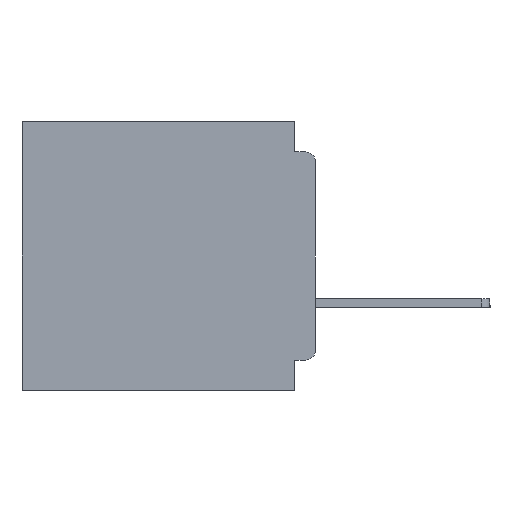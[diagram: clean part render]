
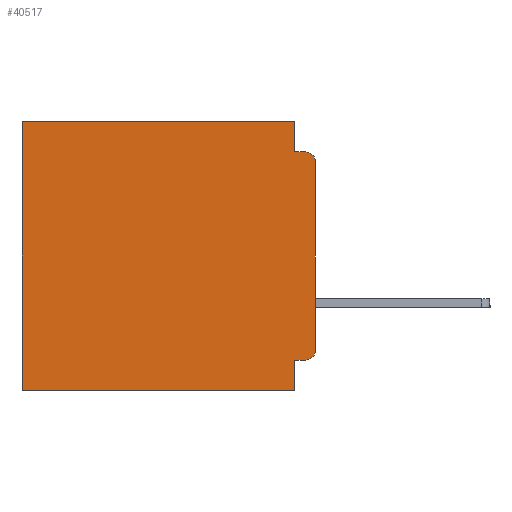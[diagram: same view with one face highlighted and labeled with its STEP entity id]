
A CAD part, left-side view. The second image highlights one B-rep face of the part: STEP entity #40517.
In plain terms, the highlighted planar face has unit normal (-1, 0, 0).
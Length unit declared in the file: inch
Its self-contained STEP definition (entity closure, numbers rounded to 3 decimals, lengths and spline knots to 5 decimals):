
#1040 = ORIENTED_EDGE ( 'NONE', *, *, #40793, .T. ) ;
#1313 = VERTEX_POINT ( 'NONE', #37785 ) ;
#1515 = LINE ( 'NONE', #48837, #16003 ) ;
#2371 = CARTESIAN_POINT ( 'NONE',  ( 0.3, 0.031, -0.4 ) ) ;
#3398 = DIRECTION ( 'NONE',  ( 0., 0., -1. ) ) ;
#3695 = CARTESIAN_POINT ( 'NONE',  ( 0.3, 0., 0. ) ) ;
#3770 = VERTEX_POINT ( 'NONE', #52345 ) ;
#4352 = VECTOR ( 'NONE', #5088, 39.37008 ) ;
#4801 = CARTESIAN_POINT ( 'NONE',  ( 0.3, 0.437, -0.4 ) ) ;
#5088 = DIRECTION ( 'NONE',  ( 0., 0., -1. ) ) ;
#5142 = DIRECTION ( 'NONE',  ( 0., 1., 0. ) ) ;
#5832 = FACE_OUTER_BOUND ( 'NONE', #31797, .T. ) ;
#6410 = VERTEX_POINT ( 'NONE', #62724 ) ;
#6475 = EDGE_CURVE ( 'NONE', #6410, #33333, #1515, .T. ) ;
#6576 = LINE ( 'NONE', #28269, #8101 ) ;
#6905 = EDGE_CURVE ( 'NONE', #55357, #3770, #30349, .T. ) ;
#7275 = DIRECTION ( 'NONE',  ( 0., 0., -1. ) ) ;
#7650 = ORIENTED_EDGE ( 'NONE', *, *, #45252, .T. ) ;
#8101 = VECTOR ( 'NONE', #33180, 39.37008 ) ;
#8337 = VECTOR ( 'NONE', #45586, 39.37008 ) ;
#8449 = VERTEX_POINT ( 'NONE', #25934 ) ;
#9834 = PLANE ( 'NONE',  #43445 ) ;
#10228 = AXIS2_PLACEMENT_3D ( 'NONE', #61396, #32515, #3398 ) ;
#11049 = LINE ( 'NONE', #2371, #35330 ) ;
#11069 = VERTEX_POINT ( 'NONE', #22094 ) ;
#11484 = CARTESIAN_POINT ( 'NONE',  ( 0.3, 0., -0.045 ) ) ;
#12932 = ORIENTED_EDGE ( 'NONE', *, *, #59811, .F. ) ;
#13053 = LINE ( 'NONE', #4801, #61443 ) ;
#13683 = VERTEX_POINT ( 'NONE', #48905 ) ;
#14359 = ORIENTED_EDGE ( 'NONE', *, *, #6475, .F. ) ;
#16003 = VECTOR ( 'NONE', #5142, 39.37008 ) ;
#18357 = CARTESIAN_POINT ( 'NONE',  ( 0.3, 0., -0.06 ) ) ;
#18489 = ORIENTED_EDGE ( 'NONE', *, *, #38841, .F. ) ;
#19050 = ORIENTED_EDGE ( 'NONE', *, *, #56687, .T. ) ;
#19526 = CIRCLE ( 'NONE', #35802, 0.015 ) ;
#21776 = EDGE_CURVE ( 'NONE', #55357, #8449, #51978, .T. ) ;
#22094 = CARTESIAN_POINT ( 'NONE',  ( 0.3, 0.031, 0. ) ) ;
#24625 = DIRECTION ( 'NONE',  ( 1., 0., 0. ) ) ;
#25934 = CARTESIAN_POINT ( 'NONE',  ( 0.3, 0.031, -0.355 ) ) ;
#26228 = VECTOR ( 'NONE', #41448, 39.37008 ) ;
#26703 = DIRECTION ( 'NONE',  ( -1., 0., 0. ) ) ;
#27546 = EDGE_CURVE ( 'NONE', #1313, #52944, #58303, .T. ) ;
#28269 = CARTESIAN_POINT ( 'NONE',  ( 0.3, 0.031, 0. ) ) ;
#30239 = LINE ( 'NONE', #48576, #4352 ) ;
#30349 = CIRCLE ( 'NONE', #10228, 0.015 ) ;
#31797 = EDGE_LOOP ( 'NONE', ( #18489, #1040, #62431, #36083, #7650, #19050, #14359, #12932, #50887, #52371 ) ) ;
#32515 = DIRECTION ( 'NONE',  ( -1., 0., 0. ) ) ;
#33180 = DIRECTION ( 'NONE',  ( 0., 0., -1. ) ) ;
#33190 = CARTESIAN_POINT ( 'NONE',  ( 0.3, 0.437, -0.4 ) ) ;
#33333 = VERTEX_POINT ( 'NONE', #33190 ) ;
#35330 = VECTOR ( 'NONE', #7275, 39.37008 ) ;
#35802 = AXIS2_PLACEMENT_3D ( 'NONE', #55720, #26703, #60541 ) ;
#36083 = ORIENTED_EDGE ( 'NONE', *, *, #54011, .F. ) ;
#36593 = CARTESIAN_POINT ( 'NONE',  ( 0.3, 0., -0.355 ) ) ;
#37785 = CARTESIAN_POINT ( 'NONE',  ( 0.3, 0.031, -0.045 ) ) ;
#38090 = CARTESIAN_POINT ( 'NONE',  ( 0.3, 0.015, -0.355 ) ) ;
#38348 = CARTESIAN_POINT ( 'NONE',  ( 0.3, 0.015, -0.045 ) ) ;
#38841 = EDGE_CURVE ( 'NONE', #55961, #3770, #30239, .T. ) ;
#40517 = ADVANCED_FACE ( 'NONE', ( #5832 ), #9834, .F. ) ;
#40793 = EDGE_CURVE ( 'NONE', #55961, #52944, #19526, .T. ) ;
#41448 = DIRECTION ( 'NONE',  ( 0., 1., 0. ) ) ;
#41710 = VECTOR ( 'NONE', #47367, 39.37008 ) ;
#43445 = AXIS2_PLACEMENT_3D ( 'NONE', #53623, #24625, #58462 ) ;
#45252 = EDGE_CURVE ( 'NONE', #11069, #13683, #54545, .T. ) ;
#45586 = DIRECTION ( 'NONE',  ( 0., -1., 0. ) ) ;
#47367 = DIRECTION ( 'NONE',  ( 0., 1., 0. ) ) ;
#48506 = DIRECTION ( 'NONE',  ( 0., 0., -1. ) ) ;
#48576 = CARTESIAN_POINT ( 'NONE',  ( 0.3, 0., -0.4 ) ) ;
#48837 = CARTESIAN_POINT ( 'NONE',  ( 0.3, 0., -0.4 ) ) ;
#48905 = CARTESIAN_POINT ( 'NONE',  ( 0.3, 0.437, 0. ) ) ;
#50887 = ORIENTED_EDGE ( 'NONE', *, *, #21776, .F. ) ;
#51978 = LINE ( 'NONE', #36593, #26228 ) ;
#52345 = CARTESIAN_POINT ( 'NONE',  ( 0.3, 0., -0.34 ) ) ;
#52371 = ORIENTED_EDGE ( 'NONE', *, *, #6905, .T. ) ;
#52944 = VERTEX_POINT ( 'NONE', #38348 ) ;
#53623 = CARTESIAN_POINT ( 'NONE',  ( 0.3, 0., -0.4 ) ) ;
#54011 = EDGE_CURVE ( 'NONE', #11069, #1313, #6576, .T. ) ;
#54545 = LINE ( 'NONE', #3695, #41710 ) ;
#55357 = VERTEX_POINT ( 'NONE', #38090 ) ;
#55720 = CARTESIAN_POINT ( 'NONE',  ( 0.3, 0.015, -0.06 ) ) ;
#55961 = VERTEX_POINT ( 'NONE', #18357 ) ;
#56687 = EDGE_CURVE ( 'NONE', #13683, #33333, #13053, .T. ) ;
#58303 = LINE ( 'NONE', #11484, #8337 ) ;
#58462 = DIRECTION ( 'NONE',  ( 0., 0., -1. ) ) ;
#59811 = EDGE_CURVE ( 'NONE', #8449, #6410, #11049, .T. ) ;
#60541 = DIRECTION ( 'NONE',  ( 0., 0., -1. ) ) ;
#61396 = CARTESIAN_POINT ( 'NONE',  ( 0.3, 0.015, -0.34 ) ) ;
#61443 = VECTOR ( 'NONE', #48506, 39.37008 ) ;
#62431 = ORIENTED_EDGE ( 'NONE', *, *, #27546, .F. ) ;
#62724 = CARTESIAN_POINT ( 'NONE',  ( 0.3, 0.031, -0.4 ) ) ;
